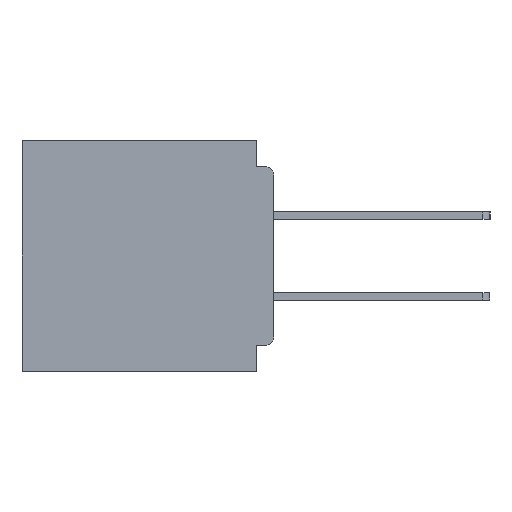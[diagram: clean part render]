
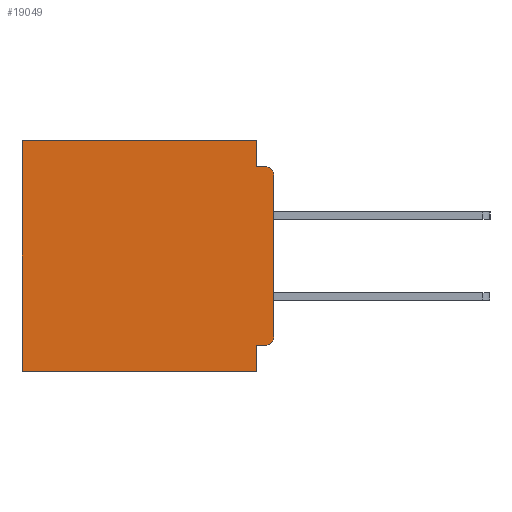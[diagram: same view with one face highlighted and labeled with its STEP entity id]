
A CAD part, left-side view. The second image highlights one B-rep face of the part: STEP entity #19049.
In plain terms, the highlighted planar face has unit normal (-1, 0, 0).
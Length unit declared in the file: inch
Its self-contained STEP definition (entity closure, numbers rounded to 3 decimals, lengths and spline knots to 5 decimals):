
#268 = LINE ( 'NONE', #21576, #8383 ) ;
#723 = ORIENTED_EDGE ( 'NONE', *, *, #42840, .F. ) ;
#1997 = ORIENTED_EDGE ( 'NONE', *, *, #9682, .F. ) ;
#2567 = CARTESIAN_POINT ( 'NONE',  ( 0.3, 0., -0.355 ) ) ;
#3100 = DIRECTION ( 'NONE',  ( 0., 0., -1. ) ) ;
#3457 = DIRECTION ( 'NONE',  ( 0., 0., -1. ) ) ;
#3582 = VERTEX_POINT ( 'NONE', #43807 ) ;
#4282 = VECTOR ( 'NONE', #5526, 39.37008 ) ;
#5183 = DIRECTION ( 'NONE',  ( 0., 1., 0. ) ) ;
#5526 = DIRECTION ( 'NONE',  ( 0., -1., 0. ) ) ;
#5742 = CARTESIAN_POINT ( 'NONE',  ( 0.3, 0.031, -0.4 ) ) ;
#7045 = VECTOR ( 'NONE', #40901, 39.37008 ) ;
#7161 = VECTOR ( 'NONE', #5183, 39.37008 ) ;
#7166 = EDGE_CURVE ( 'NONE', #3582, #36566, #34234, .T. ) ;
#7767 = DIRECTION ( 'NONE',  ( 0., 0., -1. ) ) ;
#8383 = VECTOR ( 'NONE', #7767, 39.37008 ) ;
#8924 = LINE ( 'NONE', #10411, #44970 ) ;
#9013 = ORIENTED_EDGE ( 'NONE', *, *, #16184, .T. ) ;
#9545 = CARTESIAN_POINT ( 'NONE',  ( 0.3, 0.015, -0.34 ) ) ;
#9682 = EDGE_CURVE ( 'NONE', #10986, #17562, #10421, .T. ) ;
#9747 = CARTESIAN_POINT ( 'NONE',  ( 0.3, 0.031, -0.355 ) ) ;
#10411 = CARTESIAN_POINT ( 'NONE',  ( 0.3, 0.031, 0. ) ) ;
#10421 = LINE ( 'NONE', #2567, #17488 ) ;
#10644 = CARTESIAN_POINT ( 'NONE',  ( 0.3, 0., -0.06 ) ) ;
#10936 = VERTEX_POINT ( 'NONE', #10644 ) ;
#10986 = VERTEX_POINT ( 'NONE', #42375 ) ;
#11752 = CARTESIAN_POINT ( 'NONE',  ( 0.3, 0.015, -0.045 ) ) ;
#12888 = ORIENTED_EDGE ( 'NONE', *, *, #38139, .F. ) ;
#12966 = CARTESIAN_POINT ( 'NONE',  ( 0.3, 0., -0.4 ) ) ;
#13036 = DIRECTION ( 'NONE',  ( 0., 0., -1. ) ) ;
#13326 = EDGE_CURVE ( 'NONE', #10936, #36566, #31939, .T. ) ;
#14429 = EDGE_LOOP ( 'NONE', ( #723, #38475, #33483, #23921, #9013, #23323, #12888, #19731, #1997, #17111 ) ) ;
#14724 = EDGE_CURVE ( 'NONE', #22928, #3582, #8924, .T. ) ;
#15043 = VECTOR ( 'NONE', #3457, 39.37008 ) ;
#15442 = VECTOR ( 'NONE', #30081, 39.37008 ) ;
#15461 = CARTESIAN_POINT ( 'NONE',  ( 0.3, 0., 0. ) ) ;
#15978 = VERTEX_POINT ( 'NONE', #42545 ) ;
#16167 = LINE ( 'NONE', #38345, #15043 ) ;
#16184 = EDGE_CURVE ( 'NONE', #22928, #29523, #26711, .T. ) ;
#16459 = VERTEX_POINT ( 'NONE', #20653 ) ;
#17111 = ORIENTED_EDGE ( 'NONE', *, *, #18118, .T. ) ;
#17488 = VECTOR ( 'NONE', #19921, 39.37008 ) ;
#17562 = VERTEX_POINT ( 'NONE', #9747 ) ;
#17819 = CIRCLE ( 'NONE', #30381, 0.015 ) ;
#18118 = EDGE_CURVE ( 'NONE', #10986, #25228, #17819, .T. ) ;
#18895 = DIRECTION ( 'NONE',  ( 1., 0., 0. ) ) ;
#19049 = ADVANCED_FACE ( 'NONE', ( #27625 ), #39830, .F. ) ;
#19731 = ORIENTED_EDGE ( 'NONE', *, *, #44384, .F. ) ;
#19921 = DIRECTION ( 'NONE',  ( 0., 1., 0. ) ) ;
#20653 = CARTESIAN_POINT ( 'NONE',  ( 0.3, 0.031, -0.4 ) ) ;
#21576 = CARTESIAN_POINT ( 'NONE',  ( 0.3, 0.437, -0.4 ) ) ;
#22562 = EDGE_CURVE ( 'NONE', #29523, #15978, #268, .T. ) ;
#22823 = CARTESIAN_POINT ( 'NONE',  ( 0.3, 0., -0.045 ) ) ;
#22928 = VERTEX_POINT ( 'NONE', #44641 ) ;
#23323 = ORIENTED_EDGE ( 'NONE', *, *, #22562, .T. ) ;
#23900 = DIRECTION ( 'NONE',  ( -1., 0., 0. ) ) ;
#23921 = ORIENTED_EDGE ( 'NONE', *, *, #14724, .F. ) ;
#25228 = VERTEX_POINT ( 'NONE', #37583 ) ;
#26711 = LINE ( 'NONE', #15461, #7161 ) ;
#27625 = FACE_OUTER_BOUND ( 'NONE', #14429, .T. ) ;
#29253 = CARTESIAN_POINT ( 'NONE',  ( 0.3, 0., -0.4 ) ) ;
#29523 = VERTEX_POINT ( 'NONE', #45023 ) ;
#30081 = DIRECTION ( 'NONE',  ( 0., 0., -1. ) ) ;
#30381 = AXIS2_PLACEMENT_3D ( 'NONE', #9545, #33929, #13036 ) ;
#31593 = AXIS2_PLACEMENT_3D ( 'NONE', #29253, #18895, #43366 ) ;
#31939 = CIRCLE ( 'NONE', #37277, 0.015 ) ;
#33483 = ORIENTED_EDGE ( 'NONE', *, *, #7166, .F. ) ;
#33929 = DIRECTION ( 'NONE',  ( -1., 0., 0. ) ) ;
#34234 = LINE ( 'NONE', #22823, #4282 ) ;
#34806 = DIRECTION ( 'NONE',  ( 0., 0., -1. ) ) ;
#34829 = LINE ( 'NONE', #12966, #7045 ) ;
#36566 = VERTEX_POINT ( 'NONE', #11752 ) ;
#37277 = AXIS2_PLACEMENT_3D ( 'NONE', #44897, #23900, #3100 ) ;
#37583 = CARTESIAN_POINT ( 'NONE',  ( 0.3, 0., -0.34 ) ) ;
#38139 = EDGE_CURVE ( 'NONE', #16459, #15978, #34829, .T. ) ;
#38345 = CARTESIAN_POINT ( 'NONE',  ( 0.3, 0., -0.4 ) ) ;
#38475 = ORIENTED_EDGE ( 'NONE', *, *, #13326, .T. ) ;
#39830 = PLANE ( 'NONE',  #31593 ) ;
#40901 = DIRECTION ( 'NONE',  ( 0., 1., 0. ) ) ;
#42257 = LINE ( 'NONE', #5742, #15442 ) ;
#42375 = CARTESIAN_POINT ( 'NONE',  ( 0.3, 0.015, -0.355 ) ) ;
#42545 = CARTESIAN_POINT ( 'NONE',  ( 0.3, 0.437, -0.4 ) ) ;
#42840 = EDGE_CURVE ( 'NONE', #10936, #25228, #16167, .T. ) ;
#43366 = DIRECTION ( 'NONE',  ( 0., 0., -1. ) ) ;
#43807 = CARTESIAN_POINT ( 'NONE',  ( 0.3, 0.031, -0.045 ) ) ;
#44384 = EDGE_CURVE ( 'NONE', #17562, #16459, #42257, .T. ) ;
#44641 = CARTESIAN_POINT ( 'NONE',  ( 0.3, 0.031, 0. ) ) ;
#44897 = CARTESIAN_POINT ( 'NONE',  ( 0.3, 0.015, -0.06 ) ) ;
#44970 = VECTOR ( 'NONE', #34806, 39.37008 ) ;
#45023 = CARTESIAN_POINT ( 'NONE',  ( 0.3, 0.437, 0. ) ) ;
